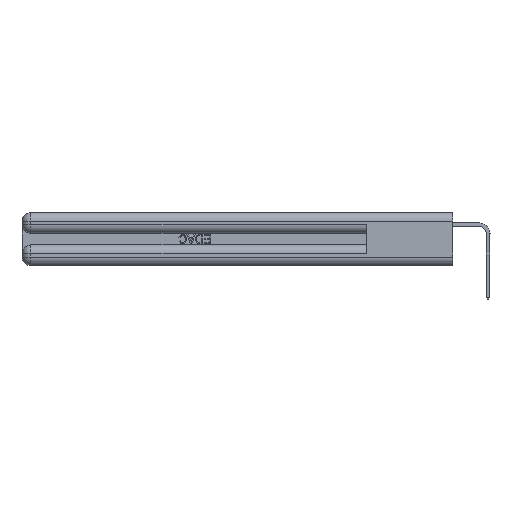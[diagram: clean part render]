
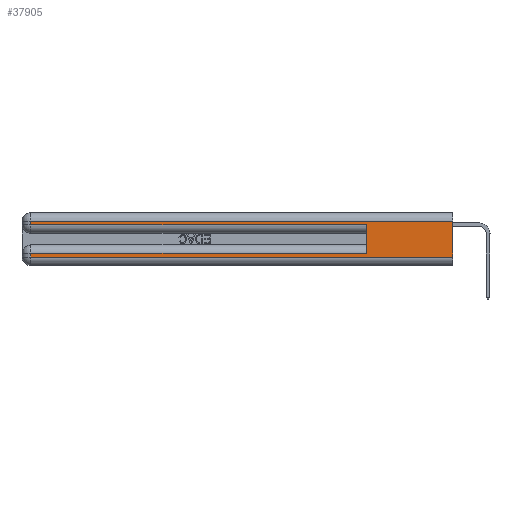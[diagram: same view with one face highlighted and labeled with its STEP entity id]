
A CAD part, left-side view. The second image highlights one B-rep face of the part: STEP entity #37905.
In plain terms, the highlighted planar face has unit normal (-1, 0, 0).
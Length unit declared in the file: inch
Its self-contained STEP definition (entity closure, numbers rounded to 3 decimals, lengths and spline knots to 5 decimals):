
#384 = CARTESIAN_POINT ( 'NONE',  ( 0., 2.94, 0.06 ) ) ;
#1054 = DIRECTION ( 'NONE',  ( 0., 1., 0. ) ) ;
#1171 = DIRECTION ( 'NONE',  ( 0., 0., -1. ) ) ;
#3526 = LINE ( 'NONE', #34640, #44725 ) ;
#3996 = VERTEX_POINT ( 'NONE', #13446 ) ;
#4043 = VERTEX_POINT ( 'NONE', #9625 ) ;
#4063 = FACE_OUTER_BOUND ( 'NONE', #19970, .T. ) ;
#4644 = VECTOR ( 'NONE', #35610, 39.37008 ) ;
#5535 = ORIENTED_EDGE ( 'NONE', *, *, #14185, .T. ) ;
#6499 = LINE ( 'NONE', #38003, #39464 ) ;
#7922 = DIRECTION ( 'NONE',  ( 0., 1., 0. ) ) ;
#7931 = CARTESIAN_POINT ( 'NONE',  ( 0., 0., 0.06 ) ) ;
#8941 = EDGE_CURVE ( 'NONE', #22645, #3996, #42504, .T. ) ;
#9254 = EDGE_CURVE ( 'NONE', #25252, #3996, #6499, .T. ) ;
#9625 = CARTESIAN_POINT ( 'NONE',  ( 0., 2.94, 0.31 ) ) ;
#10720 = VERTEX_POINT ( 'NONE', #384 ) ;
#11057 = LINE ( 'NONE', #17320, #31773 ) ;
#12038 = EDGE_CURVE ( 'NONE', #10720, #32975, #39771, .T. ) ;
#13380 = ORIENTED_EDGE ( 'NONE', *, *, #43413, .T. ) ;
#13446 = CARTESIAN_POINT ( 'NONE',  ( 0., 0.6, 0.285 ) ) ;
#14185 = EDGE_CURVE ( 'NONE', #4043, #22645, #44138, .T. ) ;
#14564 = DIRECTION ( 'NONE',  ( 1., 0., 0. ) ) ;
#15739 = ORIENTED_EDGE ( 'NONE', *, *, #12038, .T. ) ;
#16903 = LINE ( 'NONE', #47702, #4644 ) ;
#17320 = CARTESIAN_POINT ( 'NONE',  ( 0., 0., 0.085 ) ) ;
#17412 = DIRECTION ( 'NONE',  ( 0., 0., 1. ) ) ;
#19042 = CARTESIAN_POINT ( 'NONE',  ( 0., 0., 0.285 ) ) ;
#19221 = VECTOR ( 'NONE', #39821, 39.37008 ) ;
#19970 = EDGE_LOOP ( 'NONE', ( #52252, #50846, #5535, #21196, #40454, #24836, #13380, #15739 ) ) ;
#21196 = ORIENTED_EDGE ( 'NONE', *, *, #8941, .T. ) ;
#22645 = VERTEX_POINT ( 'NONE', #37842 ) ;
#23138 = CARTESIAN_POINT ( 'NONE',  ( 0., 2.94, 0.085 ) ) ;
#23949 = CARTESIAN_POINT ( 'NONE',  ( 0., 0., 0.31 ) ) ;
#24836 = ORIENTED_EDGE ( 'NONE', *, *, #43817, .T. ) ;
#25252 = VERTEX_POINT ( 'NONE', #33282 ) ;
#25956 = CARTESIAN_POINT ( 'NONE',  ( 0., 2.94, 0.37 ) ) ;
#26130 = CARTESIAN_POINT ( 'NONE',  ( 0., 0., 0.06 ) ) ;
#29168 = VERTEX_POINT ( 'NONE', #23949 ) ;
#30154 = VECTOR ( 'NONE', #30307, 39.37008 ) ;
#30307 = DIRECTION ( 'NONE',  ( 0., -1., 0. ) ) ;
#30431 = VERTEX_POINT ( 'NONE', #23138 ) ;
#31773 = VECTOR ( 'NONE', #1054, 39.37008 ) ;
#32975 = VERTEX_POINT ( 'NONE', #7931 ) ;
#33282 = CARTESIAN_POINT ( 'NONE',  ( 0., 0.6, 0.085 ) ) ;
#34498 = VECTOR ( 'NONE', #1171, 39.37008 ) ;
#34640 = CARTESIAN_POINT ( 'NONE',  ( 0., 0., 0.37 ) ) ;
#35610 = DIRECTION ( 'NONE',  ( 0., 0., -1. ) ) ;
#36846 = CARTESIAN_POINT ( 'NONE',  ( 0., 0., 0.31 ) ) ;
#36886 = AXIS2_PLACEMENT_3D ( 'NONE', #39313, #14564, #43453 ) ;
#37842 = CARTESIAN_POINT ( 'NONE',  ( 0., 2.94, 0.285 ) ) ;
#37905 = ADVANCED_FACE ( 'NONE', ( #4063 ), #39133, .F. ) ;
#38003 = CARTESIAN_POINT ( 'NONE',  ( 0., 0.6, 0.145 ) ) ;
#38769 = DIRECTION ( 'NONE',  ( 0., 0., -1. ) ) ;
#39133 = PLANE ( 'NONE',  #36886 ) ;
#39313 = CARTESIAN_POINT ( 'NONE',  ( 0., 0., 0.37 ) ) ;
#39464 = VECTOR ( 'NONE', #17412, 39.37008 ) ;
#39771 = LINE ( 'NONE', #26130, #30154 ) ;
#39821 = DIRECTION ( 'NONE',  ( 0., -1., 0. ) ) ;
#40454 = ORIENTED_EDGE ( 'NONE', *, *, #9254, .F. ) ;
#42504 = LINE ( 'NONE', #19042, #19221 ) ;
#43413 = EDGE_CURVE ( 'NONE', #30431, #10720, #16903, .T. ) ;
#43453 = DIRECTION ( 'NONE',  ( 0., 0., -1. ) ) ;
#43581 = EDGE_CURVE ( 'NONE', #29168, #4043, #51831, .T. ) ;
#43817 = EDGE_CURVE ( 'NONE', #25252, #30431, #11057, .T. ) ;
#44138 = LINE ( 'NONE', #25956, #34498 ) ;
#44725 = VECTOR ( 'NONE', #38769, 39.37008 ) ;
#47702 = CARTESIAN_POINT ( 'NONE',  ( 0., 2.94, 0.37 ) ) ;
#50527 = VECTOR ( 'NONE', #7922, 39.37008 ) ;
#50846 = ORIENTED_EDGE ( 'NONE', *, *, #43581, .T. ) ;
#51628 = EDGE_CURVE ( 'NONE', #29168, #32975, #3526, .T. ) ;
#51831 = LINE ( 'NONE', #36846, #50527 ) ;
#52252 = ORIENTED_EDGE ( 'NONE', *, *, #51628, .F. ) ;
